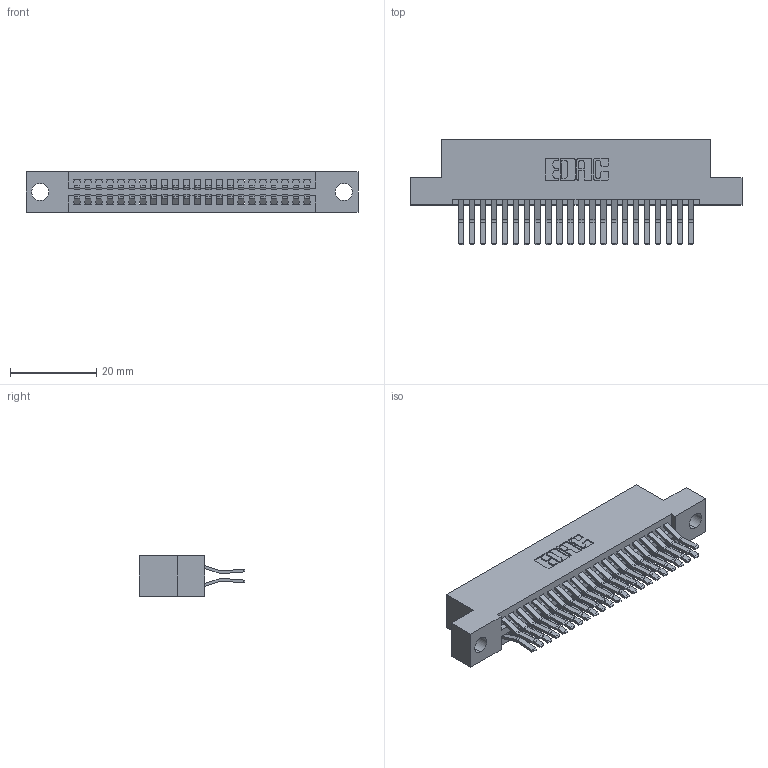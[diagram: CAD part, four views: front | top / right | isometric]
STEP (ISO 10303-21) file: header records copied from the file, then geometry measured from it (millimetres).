
FILE_DESCRIPTION (( 'STEP AP203' ), '1' );
FILE_NAME ('345-044-560-204.STEP', '2021-05-20T02:10:05', ( '' ), ( '' ), 'SwSTEP 2.0', 'SolidWorks 2020', '' );
FILE_SCHEMA (( 'CONFIG_CONTROL_DESIGN' ));
Length unit declared in the file: inch
Products named in the file (3): 345 Part_Flush Mounting Lugs - 0.156 Dia-TI; 345-044-560-204; 345-292-001_560 Tail
Assembly tree (45 placements, depth 2):
  345-044-560-204
    345 Part_Flush Mounting Lugs - 0.156 Dia-TI
    345-292-001_560 Tail  x44
Bounding box: 77.09 x 24.45 x 9.4 mm (x, y, z)
Volume: 7485.3 mm3; surface area: 11270.5 mm2
Topology: 45 solids, 45 shells, 2428 faces, 7197 edges, 4738 vertices
Faces by surface type: plane 1546, cylinder 882
Entity records: 20461 total; most frequent: CARTESIAN_POINT 3454, ORIENTED_EDGE 3386, DIRECTION 3073, EDGE_CURVE 1693, VECTOR 1469, LINE 1469, VERTEX_POINT 1126, AXIS2_PLACEMENT_3D 802
